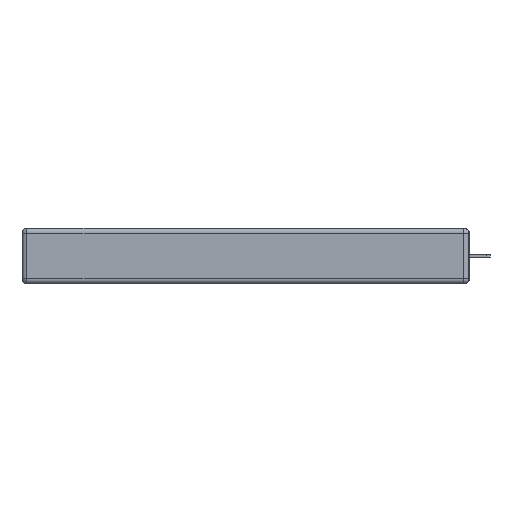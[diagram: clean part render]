
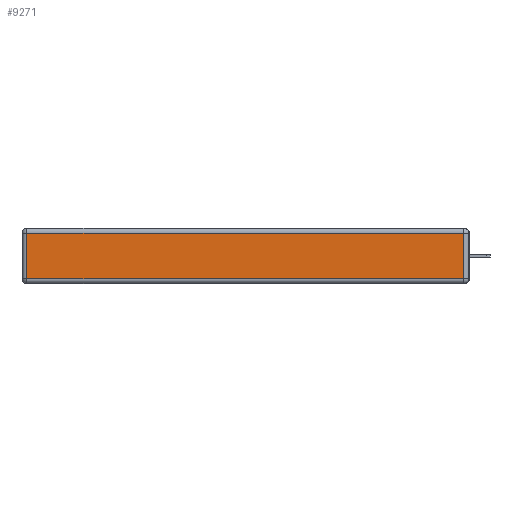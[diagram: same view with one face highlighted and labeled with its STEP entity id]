
A CAD part, left-side view. The second image highlights one B-rep face of the part: STEP entity #9271.
In plain terms, the highlighted planar face has unit normal (-1, 0, 0).
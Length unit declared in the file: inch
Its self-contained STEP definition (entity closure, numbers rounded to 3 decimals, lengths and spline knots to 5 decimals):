
#1645 = CARTESIAN_POINT ( 'NONE',  ( 0., 2.75, -0.03 ) ) ;
#4313 = VERTEX_POINT ( 'NONE', #11668 ) ;
#4398 = VERTEX_POINT ( 'NONE', #7414 ) ;
#4546 = VECTOR ( 'NONE', #13026, 39.37008 ) ;
#6041 = DIRECTION ( 'NONE',  ( 0., 0., 1. ) ) ;
#6674 = VECTOR ( 'NONE', #20063, 39.37008 ) ;
#7414 = CARTESIAN_POINT ( 'NONE',  ( 0., 0.03, -0.313 ) ) ;
#7598 = VERTEX_POINT ( 'NONE', #29536 ) ;
#8168 = EDGE_LOOP ( 'NONE', ( #22475, #23135, #9520, #20290 ) ) ;
#8312 = CARTESIAN_POINT ( 'NONE',  ( 0., 0.03, -0.343 ) ) ;
#8719 = EDGE_CURVE ( 'NONE', #4398, #22055, #28975, .T. ) ;
#9234 = CARTESIAN_POINT ( 'NONE',  ( 0., 0.03, -0.03 ) ) ;
#9271 = ADVANCED_FACE ( 'NONE', ( #22986 ), #22832, .T. ) ;
#9520 = ORIENTED_EDGE ( 'NONE', *, *, #28927, .T. ) ;
#11668 = CARTESIAN_POINT ( 'NONE',  ( 0., 2.72, -0.313 ) ) ;
#13026 = DIRECTION ( 'NONE',  ( 0., 0., -1. ) ) ;
#14818 = EDGE_CURVE ( 'NONE', #4313, #4398, #26729, .T. ) ;
#15370 = LINE ( 'NONE', #1645, #6674 ) ;
#15687 = CARTESIAN_POINT ( 'NONE',  ( 0., 0., -0.313 ) ) ;
#16687 = VECTOR ( 'NONE', #6041, 39.37008 ) ;
#19603 = EDGE_CURVE ( 'NONE', #7598, #4313, #29606, .T. ) ;
#20063 = DIRECTION ( 'NONE',  ( 0., 1., 0. ) ) ;
#20290 = ORIENTED_EDGE ( 'NONE', *, *, #19603, .T. ) ;
#22055 = VERTEX_POINT ( 'NONE', #9234 ) ;
#22475 = ORIENTED_EDGE ( 'NONE', *, *, #14818, .T. ) ;
#22488 = DIRECTION ( 'NONE',  ( 0., -1., 0. ) ) ;
#22832 = PLANE ( 'NONE',  #22998 ) ;
#22986 = FACE_OUTER_BOUND ( 'NONE', #8168, .T. ) ;
#22998 = AXIS2_PLACEMENT_3D ( 'NONE', #27675, #25377, #25089 ) ;
#23135 = ORIENTED_EDGE ( 'NONE', *, *, #8719, .T. ) ;
#24598 = VECTOR ( 'NONE', #22488, 39.37008 ) ;
#25056 = CARTESIAN_POINT ( 'NONE',  ( 0., 2.72, -0.343 ) ) ;
#25089 = DIRECTION ( 'NONE',  ( 0., 0., 1. ) ) ;
#25377 = DIRECTION ( 'NONE',  ( -1., 0., 0. ) ) ;
#26729 = LINE ( 'NONE', #15687, #24598 ) ;
#27675 = CARTESIAN_POINT ( 'NONE',  ( 0., 0., -0.343 ) ) ;
#28927 = EDGE_CURVE ( 'NONE', #22055, #7598, #15370, .T. ) ;
#28975 = LINE ( 'NONE', #8312, #16687 ) ;
#29536 = CARTESIAN_POINT ( 'NONE',  ( 0., 2.72, -0.03 ) ) ;
#29606 = LINE ( 'NONE', #25056, #4546 ) ;
